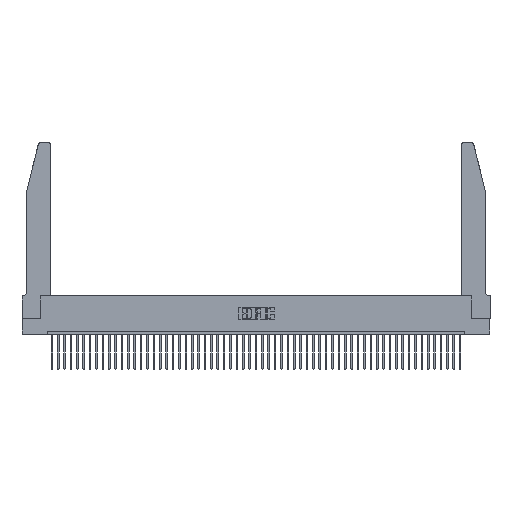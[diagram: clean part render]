
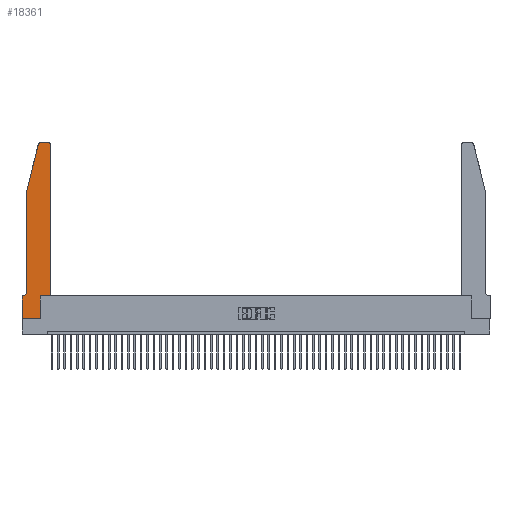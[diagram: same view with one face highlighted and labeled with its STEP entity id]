
A CAD part, top view. The second image highlights one B-rep face of the part: STEP entity #18361.
In plain terms, the highlighted planar face has unit normal (0, 0, 1).
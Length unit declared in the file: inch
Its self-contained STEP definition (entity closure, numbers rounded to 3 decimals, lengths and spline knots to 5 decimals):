
#344 = VERTEX_POINT ( 'NONE', #4578 ) ;
#1303 = CARTESIAN_POINT ( 'NONE',  ( 0., 0.35, 0.37 ) ) ;
#1367 = EDGE_CURVE ( 'NONE', #344, #34049, #48128, .T. ) ;
#1826 = CARTESIAN_POINT ( 'NONE',  ( 0., 0., 0.37 ) ) ;
#1860 = EDGE_CURVE ( 'NONE', #3060, #40836, #30352, .T. ) ;
#2409 = CARTESIAN_POINT ( 'NONE',  ( 0.2865, 0.35, 0.37 ) ) ;
#2986 = CARTESIAN_POINT ( 'NONE',  ( 0.0755, 0.35, 0.37 ) ) ;
#3060 = VERTEX_POINT ( 'NONE', #25590 ) ;
#3166 = DIRECTION ( 'NONE',  ( 1., 0., 0. ) ) ;
#3287 = AXIS2_PLACEMENT_3D ( 'NONE', #50124, #50452, #7779 ) ;
#4578 = CARTESIAN_POINT ( 'NONE',  ( 0.2865, 0., 0.37 ) ) ;
#4895 = CARTESIAN_POINT ( 'NONE',  ( 0.0755, 2., 0.37 ) ) ;
#5374 = EDGE_CURVE ( 'NONE', #47572, #23377, #36714, .T. ) ;
#5477 = CARTESIAN_POINT ( 'NONE',  ( 0.4205, 2.75, 0.37 ) ) ;
#5523 = CARTESIAN_POINT ( 'NONE',  ( 0., 0., 0.37 ) ) ;
#5524 = DIRECTION ( 'NONE',  ( -0.239, -0.971, 0. ) ) ;
#5715 = VECTOR ( 'NONE', #50130, 39.37008 ) ;
#6287 = LINE ( 'NONE', #2986, #9336 ) ;
#6704 = LINE ( 'NONE', #12563, #45833 ) ;
#6757 = DIRECTION ( 'NONE',  ( 0., 1., 0. ) ) ;
#7041 = VECTOR ( 'NONE', #8614, 39.37008 ) ;
#7244 = ORIENTED_EDGE ( 'NONE', *, *, #22877, .T. ) ;
#7779 = DIRECTION ( 'NONE',  ( 1., 0., 0. ) ) ;
#7819 = VERTEX_POINT ( 'NONE', #30511 ) ;
#8157 = EDGE_CURVE ( 'NONE', #36528, #47572, #6704, .T. ) ;
#8370 = EDGE_CURVE ( 'NONE', #23377, #32463, #17621, .T. ) ;
#8614 = DIRECTION ( 'NONE',  ( 1., 0., 0. ) ) ;
#8950 = ORIENTED_EDGE ( 'NONE', *, *, #16259, .T. ) ;
#9143 = PLANE ( 'NONE',  #26049 ) ;
#9336 = VECTOR ( 'NONE', #42458, 39.37008 ) ;
#10359 = CARTESIAN_POINT ( 'NONE',  ( 0.4505, 0.35, 0.37 ) ) ;
#11752 = LINE ( 'NONE', #11980, #42351 ) ;
#11980 = CARTESIAN_POINT ( 'NONE',  ( 0.4505, 0.35, 0.37 ) ) ;
#12563 = CARTESIAN_POINT ( 'NONE',  ( 0.0755, 2., 0.37 ) ) ;
#12670 = VECTOR ( 'NONE', #39101, 39.37008 ) ;
#13223 = EDGE_CURVE ( 'NONE', #34049, #38514, #11752, .T. ) ;
#13384 = DIRECTION ( 'NONE',  ( 1., 0., 0. ) ) ;
#13655 = ORIENTED_EDGE ( 'NONE', *, *, #5374, .T. ) ;
#13913 = VECTOR ( 'NONE', #17689, 39.37008 ) ;
#14352 = CARTESIAN_POINT ( 'NONE',  ( 0.0755, 0.42, 0.37 ) ) ;
#14612 = ORIENTED_EDGE ( 'NONE', *, *, #8157, .T. ) ;
#14933 = CARTESIAN_POINT ( 'NONE',  ( 0.2605, 2.75, 0.37 ) ) ;
#15060 = CARTESIAN_POINT ( 'NONE',  ( 0.284, 2.72, 0.37 ) ) ;
#16259 = EDGE_CURVE ( 'NONE', #38514, #3060, #26587, .T. ) ;
#16438 = VECTOR ( 'NONE', #33428, 39.37008 ) ;
#17490 = CARTESIAN_POINT ( 'NONE',  ( 0.25487, 2.72718, 0.37 ) ) ;
#17621 = CIRCLE ( 'NONE', #37897, 0.07 ) ;
#17689 = DIRECTION ( 'NONE',  ( 0., 1., 0. ) ) ;
#18307 = DIRECTION ( 'NONE',  ( 0., 0., 1. ) ) ;
#18361 = ADVANCED_FACE ( 'NONE', ( #36786 ), #9143, .T. ) ;
#19227 = CARTESIAN_POINT ( 'NONE',  ( 0.284, 2.75, 0.37 ) ) ;
#22322 = ORIENTED_EDGE ( 'NONE', *, *, #13223, .T. ) ;
#22877 = EDGE_CURVE ( 'NONE', #30664, #36528, #27305, .T. ) ;
#23322 = CARTESIAN_POINT ( 'NONE',  ( 0.0055, 0.35, 0.37 ) ) ;
#23377 = VERTEX_POINT ( 'NONE', #14352 ) ;
#23747 = DIRECTION ( 'NONE',  ( 1., 0., 0. ) ) ;
#24917 = EDGE_CURVE ( 'NONE', #32463, #7819, #6287, .T. ) ;
#25590 = CARTESIAN_POINT ( 'NONE',  ( 0.4505, 2.72, 0.37 ) ) ;
#26049 = AXIS2_PLACEMENT_3D ( 'NONE', #1303, #36828, #13384 ) ;
#26066 = LINE ( 'NONE', #43688, #12670 ) ;
#26177 = DIRECTION ( 'NONE',  ( 0., 0., -1. ) ) ;
#26587 = LINE ( 'NONE', #10359, #29034 ) ;
#27305 = CIRCLE ( 'NONE', #36355, 0.03 ) ;
#27340 = ORIENTED_EDGE ( 'NONE', *, *, #28638, .T. ) ;
#27911 = CARTESIAN_POINT ( 'NONE',  ( 0.2865, 0.35, 0.37 ) ) ;
#28638 = EDGE_CURVE ( 'NONE', #7819, #47784, #26066, .T. ) ;
#29034 = VECTOR ( 'NONE', #6757, 39.37008 ) ;
#30034 = ORIENTED_EDGE ( 'NONE', *, *, #24917, .T. ) ;
#30352 = CIRCLE ( 'NONE', #3287, 0.03 ) ;
#30511 = CARTESIAN_POINT ( 'NONE',  ( 0., 0.35, 0.37 ) ) ;
#30664 = VERTEX_POINT ( 'NONE', #19227 ) ;
#31397 = CARTESIAN_POINT ( 'NONE',  ( 0.0755, 2., 0.37 ) ) ;
#32463 = VERTEX_POINT ( 'NONE', #23322 ) ;
#33428 = DIRECTION ( 'NONE',  ( 0., -1., 0. ) ) ;
#34049 = VERTEX_POINT ( 'NONE', #27911 ) ;
#35801 = LINE ( 'NONE', #5523, #7041 ) ;
#36355 = AXIS2_PLACEMENT_3D ( 'NONE', #15060, #18307, #3166 ) ;
#36528 = VERTEX_POINT ( 'NONE', #17490 ) ;
#36714 = LINE ( 'NONE', #4895, #16438 ) ;
#36786 = FACE_OUTER_BOUND ( 'NONE', #40640, .T. ) ;
#36828 = DIRECTION ( 'NONE',  ( 0., 0., 1. ) ) ;
#37897 = AXIS2_PLACEMENT_3D ( 'NONE', #49560, #26177, #49731 ) ;
#38514 = VERTEX_POINT ( 'NONE', #47045 ) ;
#39101 = DIRECTION ( 'NONE',  ( 0., -1., 0. ) ) ;
#40640 = EDGE_LOOP ( 'NONE', ( #42647, #7244, #14612, #13655, #42029, #30034, #27340, #49382, #47484, #22322, #8950, #42888 ) ) ;
#40836 = VERTEX_POINT ( 'NONE', #5477 ) ;
#41677 = EDGE_CURVE ( 'NONE', #47784, #344, #35801, .T. ) ;
#42029 = ORIENTED_EDGE ( 'NONE', *, *, #8370, .T. ) ;
#42351 = VECTOR ( 'NONE', #23747, 39.37008 ) ;
#42458 = DIRECTION ( 'NONE',  ( -1., 0., 0. ) ) ;
#42647 = ORIENTED_EDGE ( 'NONE', *, *, #43063, .T. ) ;
#42888 = ORIENTED_EDGE ( 'NONE', *, *, #1860, .T. ) ;
#43063 = EDGE_CURVE ( 'NONE', #40836, #30664, #46087, .T. ) ;
#43688 = CARTESIAN_POINT ( 'NONE',  ( 0., 0., 0.37 ) ) ;
#45833 = VECTOR ( 'NONE', #5524, 39.37008 ) ;
#46087 = LINE ( 'NONE', #14933, #5715 ) ;
#47045 = CARTESIAN_POINT ( 'NONE',  ( 0.4505, 0.35, 0.37 ) ) ;
#47484 = ORIENTED_EDGE ( 'NONE', *, *, #1367, .T. ) ;
#47572 = VERTEX_POINT ( 'NONE', #31397 ) ;
#47784 = VERTEX_POINT ( 'NONE', #1826 ) ;
#48128 = LINE ( 'NONE', #2409, #13913 ) ;
#49382 = ORIENTED_EDGE ( 'NONE', *, *, #41677, .T. ) ;
#49560 = CARTESIAN_POINT ( 'NONE',  ( 0.0055, 0.42, 0.37 ) ) ;
#49731 = DIRECTION ( 'NONE',  ( -1., 0., 0. ) ) ;
#50124 = CARTESIAN_POINT ( 'NONE',  ( 0.4205, 2.72, 0.37 ) ) ;
#50130 = DIRECTION ( 'NONE',  ( -1., 0., 0. ) ) ;
#50452 = DIRECTION ( 'NONE',  ( 0., 0., 1. ) ) ;
